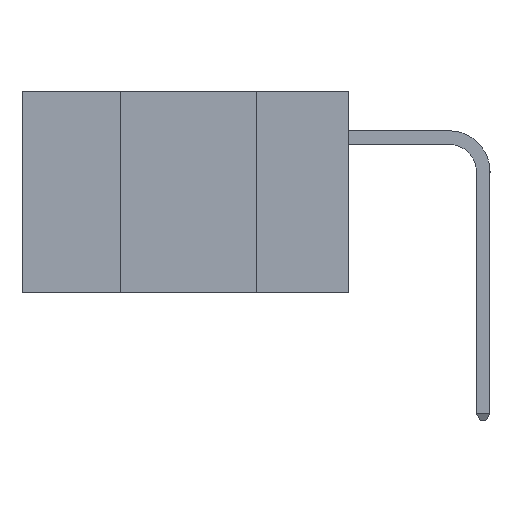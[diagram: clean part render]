
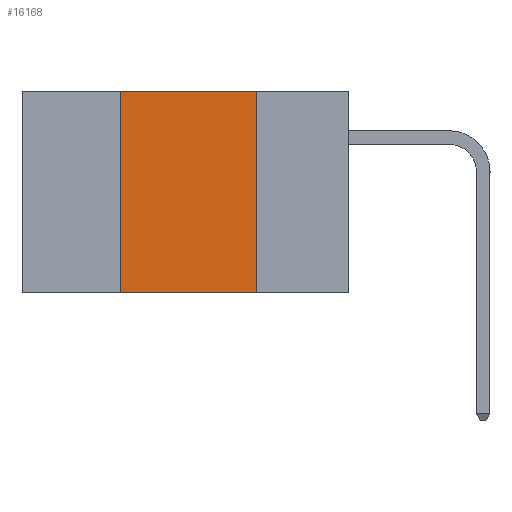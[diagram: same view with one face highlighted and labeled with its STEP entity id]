
A CAD part, left-side view. The second image highlights one B-rep face of the part: STEP entity #16168.
In plain terms, the highlighted planar face has unit normal (-1, 0, 0).
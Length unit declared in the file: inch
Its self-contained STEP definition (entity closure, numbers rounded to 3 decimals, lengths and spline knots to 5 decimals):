
#378 = CARTESIAN_POINT ( 'NONE',  ( 0., 0.17, 0. ) ) ;
#1060 = DIRECTION ( 'NONE',  ( 0., 0., -1. ) ) ;
#1112 = EDGE_CURVE ( 'NONE', #10129, #31904, #44307, .T. ) ;
#1286 = CARTESIAN_POINT ( 'NONE',  ( 0., 0.6, 0. ) ) ;
#1406 = CARTESIAN_POINT ( 'NONE',  ( 0., 0.17, 0. ) ) ;
#2228 = VERTEX_POINT ( 'NONE', #18595 ) ;
#2275 = EDGE_CURVE ( 'NONE', #2228, #10129, #29548, .T. ) ;
#3487 = ORIENTED_EDGE ( 'NONE', *, *, #19174, .F. ) ;
#3918 = ORIENTED_EDGE ( 'NONE', *, *, #2275, .F. ) ;
#5753 = CARTESIAN_POINT ( 'NONE',  ( 0., 0.42, 0. ) ) ;
#10129 = VERTEX_POINT ( 'NONE', #378 ) ;
#12988 = AXIS2_PLACEMENT_3D ( 'NONE', #1286, #22974, #1060 ) ;
#13659 = CARTESIAN_POINT ( 'NONE',  ( 0., 0.6, 0. ) ) ;
#15594 = FACE_OUTER_BOUND ( 'NONE', #18455, .T. ) ;
#15918 = ORIENTED_EDGE ( 'NONE', *, *, #1112, .F. ) ;
#16168 = ADVANCED_FACE ( 'NONE', ( #15594 ), #26776, .F. ) ;
#17904 = LINE ( 'NONE', #25277, #24981 ) ;
#18455 = EDGE_LOOP ( 'NONE', ( #15918, #3918, #3487, #45264 ) ) ;
#18595 = CARTESIAN_POINT ( 'NONE',  ( 0., 0.42, 0. ) ) ;
#18684 = VECTOR ( 'NONE', #38861, 39.37008 ) ;
#19174 = EDGE_CURVE ( 'NONE', #39041, #2228, #24339, .T. ) ;
#22974 = DIRECTION ( 'NONE',  ( 1., 0., 0. ) ) ;
#24339 = LINE ( 'NONE', #5753, #18684 ) ;
#24981 = VECTOR ( 'NONE', #29558, 39.37008 ) ;
#25277 = CARTESIAN_POINT ( 'NONE',  ( 0., 0.6, -0.37 ) ) ;
#25435 = VECTOR ( 'NONE', #26205, 39.37008 ) ;
#26205 = DIRECTION ( 'NONE',  ( 0., 0., -1. ) ) ;
#26776 = PLANE ( 'NONE',  #12988 ) ;
#29548 = LINE ( 'NONE', #13659, #40857 ) ;
#29558 = DIRECTION ( 'NONE',  ( 0., -1., 0. ) ) ;
#31904 = VERTEX_POINT ( 'NONE', #46946 ) ;
#31920 = EDGE_CURVE ( 'NONE', #39041, #31904, #17904, .T. ) ;
#35318 = DIRECTION ( 'NONE',  ( 0., -1., 0. ) ) ;
#38861 = DIRECTION ( 'NONE',  ( 0., 0., 1. ) ) ;
#39041 = VERTEX_POINT ( 'NONE', #40577 ) ;
#40577 = CARTESIAN_POINT ( 'NONE',  ( 0., 0.42, -0.37 ) ) ;
#40857 = VECTOR ( 'NONE', #35318, 39.37008 ) ;
#44307 = LINE ( 'NONE', #1406, #25435 ) ;
#45264 = ORIENTED_EDGE ( 'NONE', *, *, #31920, .T. ) ;
#46946 = CARTESIAN_POINT ( 'NONE',  ( 0., 0.17, -0.37 ) ) ;
